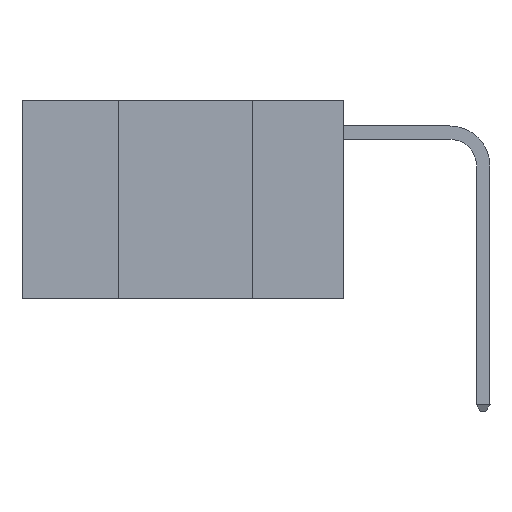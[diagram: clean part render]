
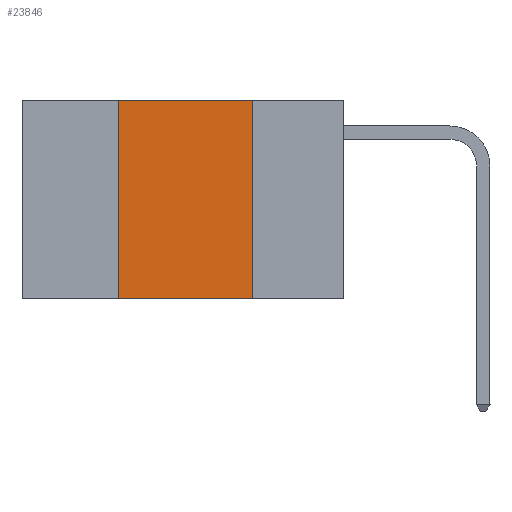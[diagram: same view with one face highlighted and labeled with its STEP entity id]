
A CAD part, left-side view. The second image highlights one B-rep face of the part: STEP entity #23846.
In plain terms, the highlighted planar face has unit normal (-1, 0, 0).
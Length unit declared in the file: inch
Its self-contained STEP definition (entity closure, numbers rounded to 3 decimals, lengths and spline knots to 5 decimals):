
#160 = DIRECTION ( 'NONE',  ( 0., -1., 0. ) ) ;
#615 = CARTESIAN_POINT ( 'NONE',  ( 0., 0.17, 0. ) ) ;
#1076 = CARTESIAN_POINT ( 'NONE',  ( 0., 0.6, 0. ) ) ;
#1321 = LINE ( 'NONE', #18781, #25056 ) ;
#1476 = EDGE_CURVE ( 'NONE', #25315, #14155, #28090, .T. ) ;
#3685 = AXIS2_PLACEMENT_3D ( 'NONE', #13228, #24607, #10926 ) ;
#4664 = LINE ( 'NONE', #24127, #22312 ) ;
#5132 = CARTESIAN_POINT ( 'NONE',  ( 0., 0.17, 0. ) ) ;
#5785 = DIRECTION ( 'NONE',  ( 0., 0., 1. ) ) ;
#6305 = VERTEX_POINT ( 'NONE', #13544 ) ;
#6425 = LINE ( 'NONE', #1076, #11906 ) ;
#6713 = VECTOR ( 'NONE', #23698, 39.37008 ) ;
#8529 = ORIENTED_EDGE ( 'NONE', *, *, #1476, .F. ) ;
#8599 = PLANE ( 'NONE',  #3685 ) ;
#9306 = ORIENTED_EDGE ( 'NONE', *, *, #11235, .F. ) ;
#10926 = DIRECTION ( 'NONE',  ( 0., 0., -1. ) ) ;
#11235 = EDGE_CURVE ( 'NONE', #15182, #6305, #4664, .T. ) ;
#11652 = CARTESIAN_POINT ( 'NONE',  ( 0., 0.42, -0.37 ) ) ;
#11906 = VECTOR ( 'NONE', #15176, 39.37008 ) ;
#13228 = CARTESIAN_POINT ( 'NONE',  ( 0., 0.6, 0. ) ) ;
#13544 = CARTESIAN_POINT ( 'NONE',  ( 0., 0.42, 0. ) ) ;
#14055 = FACE_OUTER_BOUND ( 'NONE', #26237, .T. ) ;
#14155 = VERTEX_POINT ( 'NONE', #17321 ) ;
#15176 = DIRECTION ( 'NONE',  ( 0., -1., 0. ) ) ;
#15182 = VERTEX_POINT ( 'NONE', #11652 ) ;
#15526 = ORIENTED_EDGE ( 'NONE', *, *, #28291, .F. ) ;
#17321 = CARTESIAN_POINT ( 'NONE',  ( 0., 0.17, -0.37 ) ) ;
#18781 = CARTESIAN_POINT ( 'NONE',  ( 0., 0.6, -0.37 ) ) ;
#21189 = ORIENTED_EDGE ( 'NONE', *, *, #28054, .T. ) ;
#22312 = VECTOR ( 'NONE', #5785, 39.37008 ) ;
#23698 = DIRECTION ( 'NONE',  ( 0., 0., -1. ) ) ;
#23846 = ADVANCED_FACE ( 'NONE', ( #14055 ), #8599, .F. ) ;
#24127 = CARTESIAN_POINT ( 'NONE',  ( 0., 0.42, 0. ) ) ;
#24607 = DIRECTION ( 'NONE',  ( 1., 0., 0. ) ) ;
#25056 = VECTOR ( 'NONE', #160, 39.37008 ) ;
#25315 = VERTEX_POINT ( 'NONE', #5132 ) ;
#26237 = EDGE_LOOP ( 'NONE', ( #8529, #15526, #9306, #21189 ) ) ;
#28054 = EDGE_CURVE ( 'NONE', #15182, #14155, #1321, .T. ) ;
#28090 = LINE ( 'NONE', #615, #6713 ) ;
#28291 = EDGE_CURVE ( 'NONE', #6305, #25315, #6425, .T. ) ;
